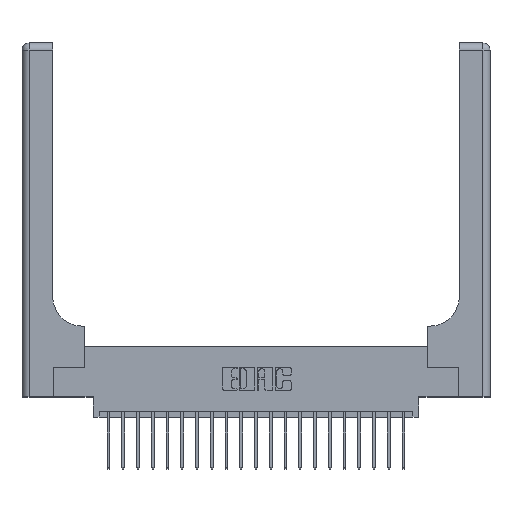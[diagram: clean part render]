
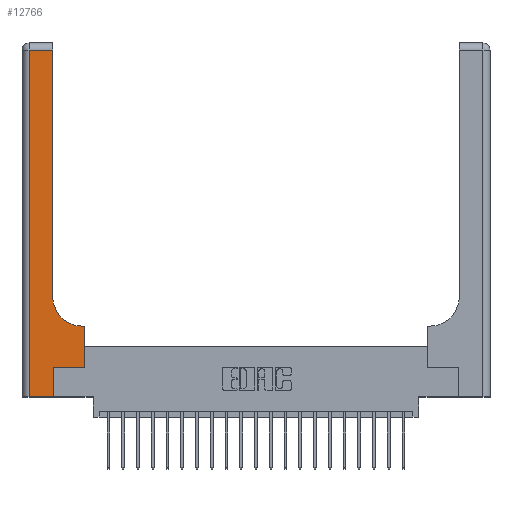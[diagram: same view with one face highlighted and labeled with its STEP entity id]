
A CAD part, top view. The second image highlights one B-rep face of the part: STEP entity #12766.
In plain terms, the highlighted planar face has unit normal (0, 0, 1).
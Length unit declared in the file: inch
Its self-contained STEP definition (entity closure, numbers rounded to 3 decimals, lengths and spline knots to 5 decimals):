
#18 = PLANE ( 'NONE',  #275 ) ;
#275 = AXIS2_PLACEMENT_3D ( 'NONE', #6661, #10493, #20465 ) ;
#389 = VECTOR ( 'NONE', #15127, 39.37008 ) ;
#397 = LINE ( 'NONE', #20959, #7480 ) ;
#440 = DIRECTION ( 'NONE',  ( 0., 0., -1. ) ) ;
#794 = LINE ( 'NONE', #14555, #10625 ) ;
#1016 = VECTOR ( 'NONE', #21344, 39.37008 ) ;
#1395 = DIRECTION ( 'NONE',  ( 1., 0., 0. ) ) ;
#1642 = CARTESIAN_POINT ( 'NONE',  ( 0.26, 2.94, 0.37 ) ) ;
#1786 = CARTESIAN_POINT ( 'NONE',  ( 0.26, 0.6, 0.37 ) ) ;
#1811 = CARTESIAN_POINT ( 'NONE',  ( 0.06, 0., 0.37 ) ) ;
#2800 = VERTEX_POINT ( 'NONE', #21923 ) ;
#2935 = CARTESIAN_POINT ( 'NONE',  ( 0.265, 0., 0.37 ) ) ;
#3022 = EDGE_CURVE ( 'NONE', #8204, #15608, #794, .T. ) ;
#3245 = LINE ( 'NONE', #1786, #21269 ) ;
#3390 = LINE ( 'NONE', #2935, #389 ) ;
#4045 = LINE ( 'NONE', #5954, #1016 ) ;
#4237 = AXIS2_PLACEMENT_3D ( 'NONE', #19541, #440, #11039 ) ;
#4613 = CARTESIAN_POINT ( 'NONE',  ( 0.06, 2.94, 0.37 ) ) ;
#5368 = CARTESIAN_POINT ( 'NONE',  ( 0.528, 0.25, 0.37 ) ) ;
#5677 = ORIENTED_EDGE ( 'NONE', *, *, #8526, .T. ) ;
#5954 = CARTESIAN_POINT ( 'NONE',  ( 0.26, 3., 0.37 ) ) ;
#5962 = VECTOR ( 'NONE', #19217, 39.37008 ) ;
#6100 = EDGE_CURVE ( 'NONE', #19854, #21407, #15499, .T. ) ;
#6165 = CARTESIAN_POINT ( 'NONE',  ( 0.51, 0.6, 0.37 ) ) ;
#6259 = CARTESIAN_POINT ( 'NONE',  ( 0.265, 0., 0.37 ) ) ;
#6661 = CARTESIAN_POINT ( 'NONE',  ( 0., 3., 0.37 ) ) ;
#6680 = EDGE_CURVE ( 'NONE', #10168, #2800, #15768, .T. ) ;
#6683 = EDGE_CURVE ( 'NONE', #2800, #13896, #4045, .T. ) ;
#7480 = VECTOR ( 'NONE', #12358, 39.37008 ) ;
#8157 = EDGE_CURVE ( 'NONE', #21407, #20700, #15922, .T. ) ;
#8204 = VERTEX_POINT ( 'NONE', #1811 ) ;
#8526 = EDGE_CURVE ( 'NONE', #20700, #10168, #3245, .T. ) ;
#8585 = CARTESIAN_POINT ( 'NONE',  ( 0.528, 0.25, 0.37 ) ) ;
#9295 = EDGE_CURVE ( 'NONE', #15608, #19854, #3390, .T. ) ;
#9596 = ORIENTED_EDGE ( 'NONE', *, *, #6680, .T. ) ;
#10168 = VERTEX_POINT ( 'NONE', #6165 ) ;
#10199 = CARTESIAN_POINT ( 'NONE',  ( 0.265, 0.25, 0.37 ) ) ;
#10480 = CARTESIAN_POINT ( 'NONE',  ( 0.528, 0.6, 0.37 ) ) ;
#10493 = DIRECTION ( 'NONE',  ( 0., 0., -1. ) ) ;
#10625 = VECTOR ( 'NONE', #11287, 39.37008 ) ;
#11039 = DIRECTION ( 'NONE',  ( 1., 0., 0. ) ) ;
#11287 = DIRECTION ( 'NONE',  ( 1., 0., 0. ) ) ;
#12358 = DIRECTION ( 'NONE',  ( -1., 0., 0. ) ) ;
#12506 = EDGE_CURVE ( 'NONE', #13896, #17667, #397, .T. ) ;
#12766 = ADVANCED_FACE ( 'NONE', ( #13554 ), #18, .F. ) ;
#13554 = FACE_OUTER_BOUND ( 'NONE', #15832, .T. ) ;
#13751 = ORIENTED_EDGE ( 'NONE', *, *, #22049, .T. ) ;
#13773 = CARTESIAN_POINT ( 'NONE',  ( 0.06, 3., 0.37 ) ) ;
#13896 = VERTEX_POINT ( 'NONE', #1642 ) ;
#14555 = CARTESIAN_POINT ( 'NONE',  ( 0., 0., 0.37 ) ) ;
#14633 = VECTOR ( 'NONE', #1395, 39.37008 ) ;
#14879 = ORIENTED_EDGE ( 'NONE', *, *, #12506, .T. ) ;
#15127 = DIRECTION ( 'NONE',  ( 0., 1., 0. ) ) ;
#15499 = LINE ( 'NONE', #10199, #14633 ) ;
#15608 = VERTEX_POINT ( 'NONE', #6259 ) ;
#15768 = CIRCLE ( 'NONE', #4237, 0.25 ) ;
#15832 = EDGE_LOOP ( 'NONE', ( #22288, #14879, #13751, #20840, #21672, #17759, #20841, #5677, #9596 ) ) ;
#15922 = LINE ( 'NONE', #8585, #5962 ) ;
#16012 = VECTOR ( 'NONE', #20573, 39.37008 ) ;
#17442 = CARTESIAN_POINT ( 'NONE',  ( 0.265, 0.25, 0.37 ) ) ;
#17667 = VERTEX_POINT ( 'NONE', #4613 ) ;
#17759 = ORIENTED_EDGE ( 'NONE', *, *, #6100, .T. ) ;
#18963 = DIRECTION ( 'NONE',  ( -1., 0., 0. ) ) ;
#19217 = DIRECTION ( 'NONE',  ( 0., 1., 0. ) ) ;
#19541 = CARTESIAN_POINT ( 'NONE',  ( 0.51, 0.85, 0.37 ) ) ;
#19854 = VERTEX_POINT ( 'NONE', #17442 ) ;
#20458 = LINE ( 'NONE', #13773, #16012 ) ;
#20465 = DIRECTION ( 'NONE',  ( -1., 0., 0. ) ) ;
#20573 = DIRECTION ( 'NONE',  ( 0., -1., 0. ) ) ;
#20700 = VERTEX_POINT ( 'NONE', #10480 ) ;
#20840 = ORIENTED_EDGE ( 'NONE', *, *, #3022, .T. ) ;
#20841 = ORIENTED_EDGE ( 'NONE', *, *, #8157, .T. ) ;
#20959 = CARTESIAN_POINT ( 'NONE',  ( 0., 2.94, 0.37 ) ) ;
#21269 = VECTOR ( 'NONE', #18963, 39.37008 ) ;
#21344 = DIRECTION ( 'NONE',  ( 0., 1., 0. ) ) ;
#21407 = VERTEX_POINT ( 'NONE', #5368 ) ;
#21672 = ORIENTED_EDGE ( 'NONE', *, *, #9295, .T. ) ;
#21923 = CARTESIAN_POINT ( 'NONE',  ( 0.26, 0.85, 0.37 ) ) ;
#22049 = EDGE_CURVE ( 'NONE', #17667, #8204, #20458, .T. ) ;
#22288 = ORIENTED_EDGE ( 'NONE', *, *, #6683, .T. ) ;
